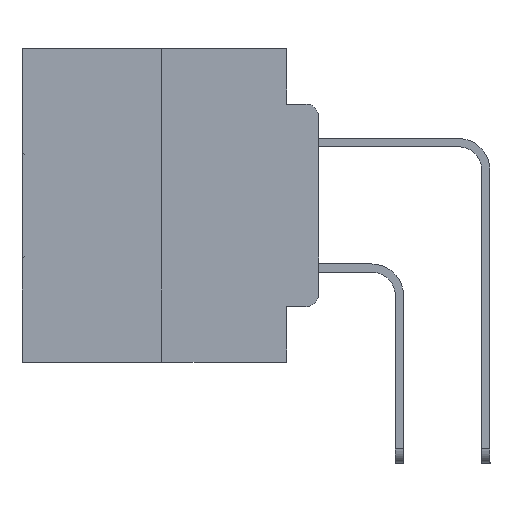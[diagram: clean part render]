
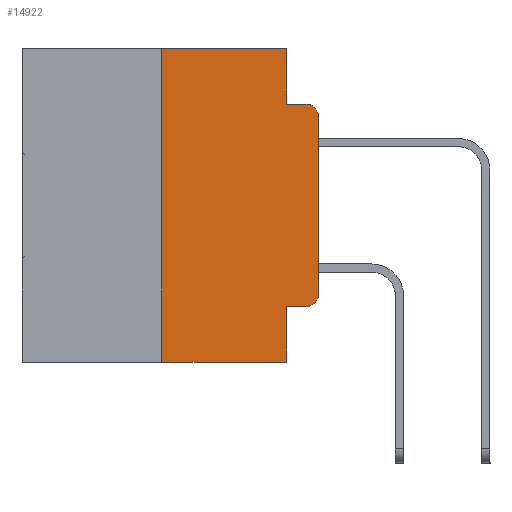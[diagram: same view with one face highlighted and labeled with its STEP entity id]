
A CAD part, left-side view. The second image highlights one B-rep face of the part: STEP entity #14922.
In plain terms, the highlighted planar face has unit normal (-1, 0, 0).
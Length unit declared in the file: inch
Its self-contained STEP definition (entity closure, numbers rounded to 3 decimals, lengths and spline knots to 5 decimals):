
#219 = CARTESIAN_POINT ( 'NONE',  ( 0., 0., -0.1085 ) ) ;
#587 = FACE_OUTER_BOUND ( 'NONE', #22783, .T. ) ;
#595 = CARTESIAN_POINT ( 'NONE',  ( 0., 0.473, 0. ) ) ;
#644 = ORIENTED_EDGE ( 'NONE', *, *, #14282, .T. ) ;
#926 = EDGE_CURVE ( 'NONE', #29025, #10924, #18599, .T. ) ;
#1036 = DIRECTION ( 'NONE',  ( 0., 0., -1. ) ) ;
#1213 = VECTOR ( 'NONE', #23227, 39.37008 ) ;
#1518 = CARTESIAN_POINT ( 'NONE',  ( 0., 0.25, 0. ) ) ;
#2007 = LINE ( 'NONE', #18253, #1213 ) ;
#2189 = VECTOR ( 'NONE', #5976, 39.37008 ) ;
#2410 = DIRECTION ( 'NONE',  ( 0., 0., -1. ) ) ;
#2470 = CARTESIAN_POINT ( 'NONE',  ( 0., 0.051, -0.4115 ) ) ;
#2594 = ORIENTED_EDGE ( 'NONE', *, *, #10792, .F. ) ;
#3938 = VECTOR ( 'NONE', #21267, 39.37008 ) ;
#4257 = CIRCLE ( 'NONE', #8785, 0.02 ) ;
#4383 = VERTEX_POINT ( 'NONE', #25443 ) ;
#4740 = VECTOR ( 'NONE', #17651, 39.37008 ) ;
#5001 = DIRECTION ( 'NONE',  ( 0., -1., 0. ) ) ;
#5099 = VERTEX_POINT ( 'NONE', #23132 ) ;
#5350 = ORIENTED_EDGE ( 'NONE', *, *, #31239, .T. ) ;
#5944 = VERTEX_POINT ( 'NONE', #9638 ) ;
#5976 = DIRECTION ( 'NONE',  ( 0., 0., 1. ) ) ;
#6061 = DIRECTION ( 'NONE',  ( 0., 0., -1. ) ) ;
#6086 = ORIENTED_EDGE ( 'NONE', *, *, #12557, .F. ) ;
#6374 = CARTESIAN_POINT ( 'NONE',  ( 0., 0.051, -0.0885 ) ) ;
#6505 = CARTESIAN_POINT ( 'NONE',  ( 0., 0.051, -0.5 ) ) ;
#8093 = DIRECTION ( 'NONE',  ( 1., 0., 0. ) ) ;
#8358 = CARTESIAN_POINT ( 'NONE',  ( 0., 0., 0. ) ) ;
#8785 = AXIS2_PLACEMENT_3D ( 'NONE', #31869, #17195, #2410 ) ;
#9320 = AXIS2_PLACEMENT_3D ( 'NONE', #595, #8093, #25343 ) ;
#9562 = ORIENTED_EDGE ( 'NONE', *, *, #27398, .T. ) ;
#9638 = CARTESIAN_POINT ( 'NONE',  ( 0., 0.25, -0.5 ) ) ;
#10622 = CARTESIAN_POINT ( 'NONE',  ( 0., 0.473, -0.5 ) ) ;
#10747 = ORIENTED_EDGE ( 'NONE', *, *, #10909, .F. ) ;
#10792 = EDGE_CURVE ( 'NONE', #14112, #31330, #2007, .T. ) ;
#10909 = EDGE_CURVE ( 'NONE', #5944, #14112, #23604, .T. ) ;
#10924 = VERTEX_POINT ( 'NONE', #6505 ) ;
#12399 = VERTEX_POINT ( 'NONE', #219 ) ;
#12557 = EDGE_CURVE ( 'NONE', #31330, #14932, #28088, .T. ) ;
#12724 = VECTOR ( 'NONE', #5001, 39.37008 ) ;
#12875 = LINE ( 'NONE', #6374, #19386 ) ;
#13077 = CARTESIAN_POINT ( 'NONE',  ( 0., 0.051, -0.0885 ) ) ;
#13469 = LINE ( 'NONE', #2470, #12724 ) ;
#14112 = VERTEX_POINT ( 'NONE', #24738 ) ;
#14282 = EDGE_CURVE ( 'NONE', #5944, #10924, #24994, .T. ) ;
#14922 = ADVANCED_FACE ( 'NONE', ( #587 ), #17889, .F. ) ;
#14932 = VERTEX_POINT ( 'NONE', #13077 ) ;
#15014 = VECTOR ( 'NONE', #6061, 39.37008 ) ;
#15169 = CARTESIAN_POINT ( 'NONE',  ( 0., 0.051, 0. ) ) ;
#15314 = LINE ( 'NONE', #8358, #2189 ) ;
#15832 = DIRECTION ( 'NONE',  ( -1., 0., 0. ) ) ;
#16875 = CIRCLE ( 'NONE', #21456, 0.02 ) ;
#17195 = DIRECTION ( 'NONE',  ( -1., 0., 0. ) ) ;
#17645 = ORIENTED_EDGE ( 'NONE', *, *, #25750, .T. ) ;
#17648 = VECTOR ( 'NONE', #25377, 39.37008 ) ;
#17651 = DIRECTION ( 'NONE',  ( 0., 0., -1. ) ) ;
#17889 = PLANE ( 'NONE',  #9320 ) ;
#18253 = CARTESIAN_POINT ( 'NONE',  ( 0., 0.473, 0. ) ) ;
#18599 = LINE ( 'NONE', #15169, #4740 ) ;
#19386 = VECTOR ( 'NONE', #21027, 39.37008 ) ;
#21027 = DIRECTION ( 'NONE',  ( 0., -1., 0. ) ) ;
#21267 = DIRECTION ( 'NONE',  ( 0., 0., 1. ) ) ;
#21456 = AXIS2_PLACEMENT_3D ( 'NONE', #30513, #15832, #1036 ) ;
#21630 = CARTESIAN_POINT ( 'NONE',  ( 0., 0., -0.3915 ) ) ;
#22702 = ORIENTED_EDGE ( 'NONE', *, *, #926, .F. ) ;
#22783 = EDGE_LOOP ( 'NONE', ( #9562, #17645, #24199, #6086, #2594, #10747, #644, #22702, #5350, #26167 ) ) ;
#23132 = CARTESIAN_POINT ( 'NONE',  ( 0., 0.02, -0.4115 ) ) ;
#23227 = DIRECTION ( 'NONE',  ( 0., -1., 0. ) ) ;
#23604 = LINE ( 'NONE', #1518, #3938 ) ;
#24108 = EDGE_CURVE ( 'NONE', #14932, #4383, #12875, .T. ) ;
#24199 = ORIENTED_EDGE ( 'NONE', *, *, #24108, .F. ) ;
#24624 = CARTESIAN_POINT ( 'NONE',  ( 0., 0.051, -0.4115 ) ) ;
#24738 = CARTESIAN_POINT ( 'NONE',  ( 0., 0.25, 0. ) ) ;
#24994 = LINE ( 'NONE', #10622, #17648 ) ;
#25030 = CARTESIAN_POINT ( 'NONE',  ( 0., 0.051, 0. ) ) ;
#25343 = DIRECTION ( 'NONE',  ( 0., 0., -1. ) ) ;
#25377 = DIRECTION ( 'NONE',  ( 0., -1., 0. ) ) ;
#25443 = CARTESIAN_POINT ( 'NONE',  ( 0., 0.02, -0.0885 ) ) ;
#25750 = EDGE_CURVE ( 'NONE', #12399, #4383, #4257, .T. ) ;
#26167 = ORIENTED_EDGE ( 'NONE', *, *, #27989, .T. ) ;
#27398 = EDGE_CURVE ( 'NONE', #28876, #12399, #15314, .T. ) ;
#27989 = EDGE_CURVE ( 'NONE', #5099, #28876, #16875, .T. ) ;
#28088 = LINE ( 'NONE', #28115, #15014 ) ;
#28115 = CARTESIAN_POINT ( 'NONE',  ( 0., 0.051, 0. ) ) ;
#28876 = VERTEX_POINT ( 'NONE', #21630 ) ;
#29025 = VERTEX_POINT ( 'NONE', #24624 ) ;
#30513 = CARTESIAN_POINT ( 'NONE',  ( 0., 0.02, -0.3915 ) ) ;
#31239 = EDGE_CURVE ( 'NONE', #29025, #5099, #13469, .T. ) ;
#31330 = VERTEX_POINT ( 'NONE', #25030 ) ;
#31869 = CARTESIAN_POINT ( 'NONE',  ( 0., 0.02, -0.1085 ) ) ;
